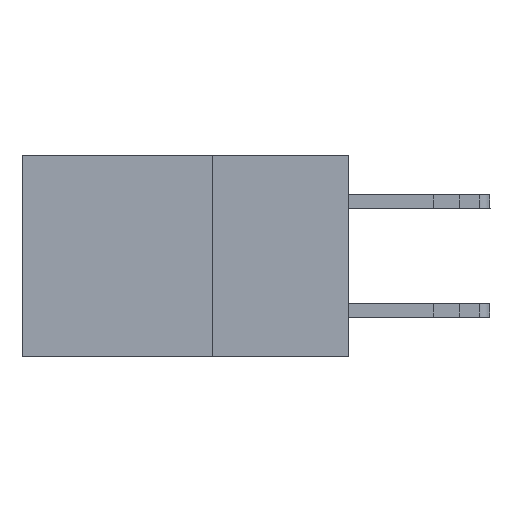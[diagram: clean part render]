
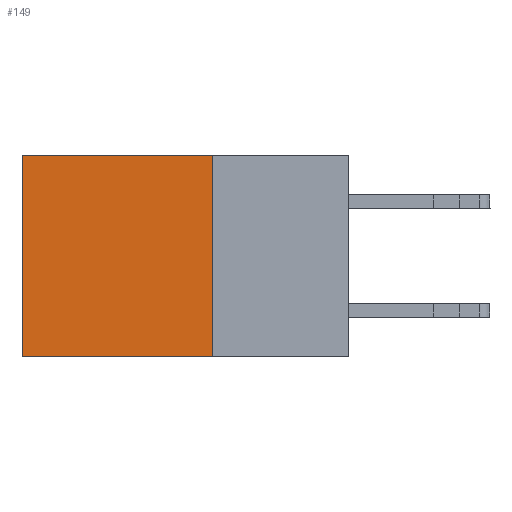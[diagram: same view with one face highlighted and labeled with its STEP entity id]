
A CAD part, left-side view. The second image highlights one B-rep face of the part: STEP entity #149.
In plain terms, the highlighted planar face has unit normal (-1, 0, 0).
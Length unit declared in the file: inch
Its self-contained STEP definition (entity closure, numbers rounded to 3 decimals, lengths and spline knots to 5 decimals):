
#149 = ADVANCED_FACE ( 'NONE', ( #12158 ), #1905, .F. ) ;
#255 = LINE ( 'NONE', #1317, #6776 ) ;
#1163 = DIRECTION ( 'NONE',  ( 0., 0., -1. ) ) ;
#1317 = CARTESIAN_POINT ( 'NONE',  ( 0.2615, 0.25, -0.37 ) ) ;
#1905 = PLANE ( 'NONE',  #5928 ) ;
#1980 = DIRECTION ( 'NONE',  ( 0., 0., -1. ) ) ;
#2271 = CARTESIAN_POINT ( 'NONE',  ( 0.2615, 0.25, -0.37 ) ) ;
#2305 = CARTESIAN_POINT ( 'NONE',  ( 0.2615, 0.25, 0. ) ) ;
#2356 = CARTESIAN_POINT ( 'NONE',  ( 0.2615, 0.25, 0. ) ) ;
#2709 = CARTESIAN_POINT ( 'NONE',  ( 0.2615, 0.6, 0. ) ) ;
#3295 = DIRECTION ( 'NONE',  ( 0., 1., 0. ) ) ;
#3438 = EDGE_CURVE ( 'NONE', #10081, #9327, #9943, .T. ) ;
#3483 = VECTOR ( 'NONE', #13091, 39.37008 ) ;
#3827 = ORIENTED_EDGE ( 'NONE', *, *, #12631, .T. ) ;
#5362 = CARTESIAN_POINT ( 'NONE',  ( 0.2615, 0.25, -0.37 ) ) ;
#5711 = CARTESIAN_POINT ( 'NONE',  ( 0.2615, 0.6, -0.37 ) ) ;
#5928 = AXIS2_PLACEMENT_3D ( 'NONE', #5362, #7669, #1980 ) ;
#6684 = VECTOR ( 'NONE', #3295, 39.37008 ) ;
#6702 = ORIENTED_EDGE ( 'NONE', *, *, #13790, .F. ) ;
#6776 = VECTOR ( 'NONE', #1163, 39.37008 ) ;
#6913 = DIRECTION ( 'NONE',  ( 0., 0., -1. ) ) ;
#7669 = DIRECTION ( 'NONE',  ( 1., 0., 0. ) ) ;
#8526 = LINE ( 'NONE', #9654, #3483 ) ;
#9155 = CARTESIAN_POINT ( 'NONE',  ( 0.2615, 0.6, -0.37 ) ) ;
#9327 = VERTEX_POINT ( 'NONE', #2709 ) ;
#9654 = CARTESIAN_POINT ( 'NONE',  ( 0.2615, 0.25, -0.37 ) ) ;
#9943 = LINE ( 'NONE', #2305, #6684 ) ;
#10081 = VERTEX_POINT ( 'NONE', #2356 ) ;
#11366 = VECTOR ( 'NONE', #6913, 39.37008 ) ;
#11381 = EDGE_CURVE ( 'NONE', #10081, #11861, #255, .T. ) ;
#11861 = VERTEX_POINT ( 'NONE', #2271 ) ;
#12158 = FACE_OUTER_BOUND ( 'NONE', #14135, .T. ) ;
#12631 = EDGE_CURVE ( 'NONE', #9327, #13217, #14758, .T. ) ;
#12732 = ORIENTED_EDGE ( 'NONE', *, *, #11381, .F. ) ;
#13091 = DIRECTION ( 'NONE',  ( 0., 1., 0. ) ) ;
#13217 = VERTEX_POINT ( 'NONE', #9155 ) ;
#13790 = EDGE_CURVE ( 'NONE', #11861, #13217, #8526, .T. ) ;
#13836 = ORIENTED_EDGE ( 'NONE', *, *, #3438, .T. ) ;
#14135 = EDGE_LOOP ( 'NONE', ( #3827, #6702, #12732, #13836 ) ) ;
#14758 = LINE ( 'NONE', #5711, #11366 ) ;
